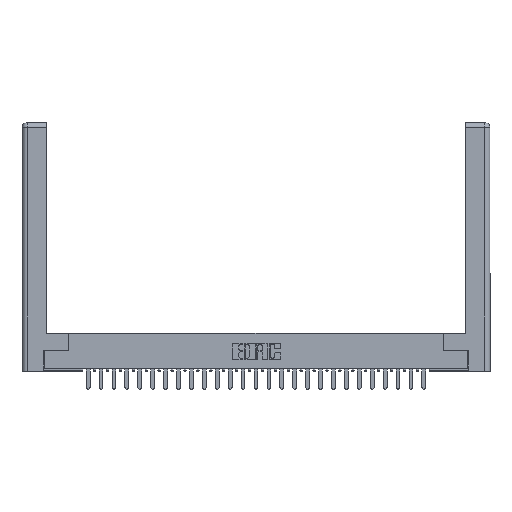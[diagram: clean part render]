
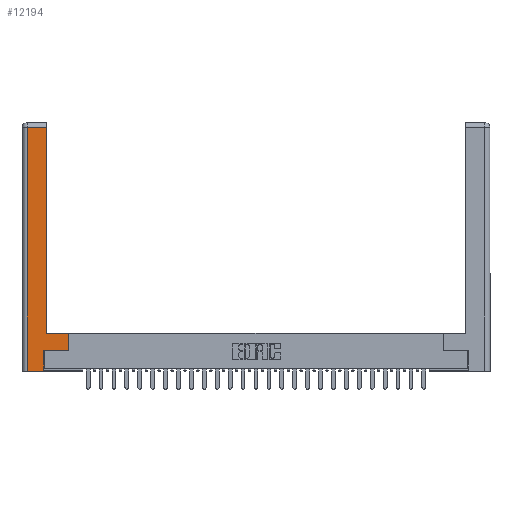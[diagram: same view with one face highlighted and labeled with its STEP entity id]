
A CAD part, top view. The second image highlights one B-rep face of the part: STEP entity #12194.
In plain terms, the highlighted planar face has unit normal (0, 0, 1).
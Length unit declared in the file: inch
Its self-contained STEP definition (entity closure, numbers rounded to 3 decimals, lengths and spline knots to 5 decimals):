
#75 = LINE ( 'NONE', #27583, #27938 ) ;
#974 = VECTOR ( 'NONE', #23557, 39.37008 ) ;
#1438 = CARTESIAN_POINT ( 'NONE',  ( 0.565, 0.45, 0. ) ) ;
#1584 = LINE ( 'NONE', #3829, #2722 ) ;
#2722 = VECTOR ( 'NONE', #24721, 39.37008 ) ;
#3088 = DIRECTION ( 'NONE',  ( 0., -1., 0. ) ) ;
#3829 = CARTESIAN_POINT ( 'NONE',  ( 0.565, 0.45, 0. ) ) ;
#4047 = CARTESIAN_POINT ( 'NONE',  ( 0., 0., 0. ) ) ;
#4332 = PLANE ( 'NONE',  #21371 ) ;
#4474 = FACE_OUTER_BOUND ( 'NONE', #8005, .T. ) ;
#4661 = EDGE_CURVE ( 'NONE', #6184, #7589, #27494, .T. ) ;
#5224 = LINE ( 'NONE', #21021, #26541 ) ;
#6061 = ORIENTED_EDGE ( 'NONE', *, *, #20825, .T. ) ;
#6083 = DIRECTION ( 'NONE',  ( -1., 0., 0. ) ) ;
#6184 = VERTEX_POINT ( 'NONE', #25987 ) ;
#6993 = DIRECTION ( 'NONE',  ( -1., 0., 0. ) ) ;
#7448 = ORIENTED_EDGE ( 'NONE', *, *, #14350, .T. ) ;
#7589 = VERTEX_POINT ( 'NONE', #17609 ) ;
#7829 = VECTOR ( 'NONE', #27779, 39.37008 ) ;
#8005 = EDGE_LOOP ( 'NONE', ( #18471, #26040, #20652, #19424, #6061, #17017, #7448, #13385 ) ) ;
#8465 = CARTESIAN_POINT ( 'NONE',  ( 0.565, 0.245, 0. ) ) ;
#10823 = DIRECTION ( 'NONE',  ( -1., 0., 0. ) ) ;
#11274 = LINE ( 'NONE', #25078, #7829 ) ;
#11750 = VERTEX_POINT ( 'NONE', #13103 ) ;
#12194 = ADVANCED_FACE ( 'NONE', ( #4474 ), #4332, .F. ) ;
#13103 = CARTESIAN_POINT ( 'NONE',  ( 0.265, 0., 0. ) ) ;
#13385 = ORIENTED_EDGE ( 'NONE', *, *, #29422, .T. ) ;
#13942 = CARTESIAN_POINT ( 'NONE',  ( 0.0615, 2.94, 0. ) ) ;
#14350 = EDGE_CURVE ( 'NONE', #28097, #17172, #1584, .T. ) ;
#14893 = VECTOR ( 'NONE', #29326, 39.37008 ) ;
#15495 = VERTEX_POINT ( 'NONE', #13942 ) ;
#16499 = CARTESIAN_POINT ( 'NONE',  ( 0.265, 0.245, 0. ) ) ;
#16721 = EDGE_CURVE ( 'NONE', #23708, #11750, #28076, .T. ) ;
#17011 = VECTOR ( 'NONE', #6083, 39.37008 ) ;
#17017 = ORIENTED_EDGE ( 'NONE', *, *, #21020, .T. ) ;
#17079 = EDGE_CURVE ( 'NONE', #15495, #23708, #25469, .T. ) ;
#17172 = VERTEX_POINT ( 'NONE', #1438 ) ;
#17609 = CARTESIAN_POINT ( 'NONE',  ( 0.295, 2.94, 0. ) ) ;
#18471 = ORIENTED_EDGE ( 'NONE', *, *, #4661, .T. ) ;
#18590 = EDGE_CURVE ( 'NONE', #7589, #15495, #75, .T. ) ;
#19186 = CARTESIAN_POINT ( 'NONE',  ( 0.265, 0., 0. ) ) ;
#19424 = ORIENTED_EDGE ( 'NONE', *, *, #16721, .T. ) ;
#20652 = ORIENTED_EDGE ( 'NONE', *, *, #17079, .T. ) ;
#20825 = EDGE_CURVE ( 'NONE', #11750, #27139, #11274, .T. ) ;
#20981 = CARTESIAN_POINT ( 'NONE',  ( 0.0615, 0., 0. ) ) ;
#21020 = EDGE_CURVE ( 'NONE', #27139, #28097, #5224, .T. ) ;
#21021 = CARTESIAN_POINT ( 'NONE',  ( 0.565, 0.245, 0. ) ) ;
#21371 = AXIS2_PLACEMENT_3D ( 'NONE', #4047, #26879, #10823 ) ;
#22695 = CARTESIAN_POINT ( 'NONE',  ( 0.295, 3., 0. ) ) ;
#23557 = DIRECTION ( 'NONE',  ( 1., 0., 0. ) ) ;
#23708 = VERTEX_POINT ( 'NONE', #27751 ) ;
#24529 = VECTOR ( 'NONE', #3088, 39.37008 ) ;
#24721 = DIRECTION ( 'NONE',  ( 0., 1., 0. ) ) ;
#24995 = LINE ( 'NONE', #29672, #17011 ) ;
#25078 = CARTESIAN_POINT ( 'NONE',  ( 0.265, 0.245, 0. ) ) ;
#25469 = LINE ( 'NONE', #20981, #24529 ) ;
#25987 = CARTESIAN_POINT ( 'NONE',  ( 0.295, 0.45, 0. ) ) ;
#26040 = ORIENTED_EDGE ( 'NONE', *, *, #18590, .T. ) ;
#26124 = DIRECTION ( 'NONE',  ( 1., 0., 0. ) ) ;
#26541 = VECTOR ( 'NONE', #26124, 39.37008 ) ;
#26879 = DIRECTION ( 'NONE',  ( 0., 0., -1. ) ) ;
#27139 = VERTEX_POINT ( 'NONE', #16499 ) ;
#27494 = LINE ( 'NONE', #22695, #14893 ) ;
#27583 = CARTESIAN_POINT ( 'NONE',  ( 0.0615, 2.94, 0. ) ) ;
#27751 = CARTESIAN_POINT ( 'NONE',  ( 0.0615, 0., 0. ) ) ;
#27779 = DIRECTION ( 'NONE',  ( 0., 1., 0. ) ) ;
#27938 = VECTOR ( 'NONE', #6993, 39.37008 ) ;
#28076 = LINE ( 'NONE', #19186, #974 ) ;
#28097 = VERTEX_POINT ( 'NONE', #8465 ) ;
#29326 = DIRECTION ( 'NONE',  ( 0., 1., 0. ) ) ;
#29422 = EDGE_CURVE ( 'NONE', #17172, #6184, #24995, .T. ) ;
#29672 = CARTESIAN_POINT ( 'NONE',  ( 0.295, 0.45, 0. ) ) ;
